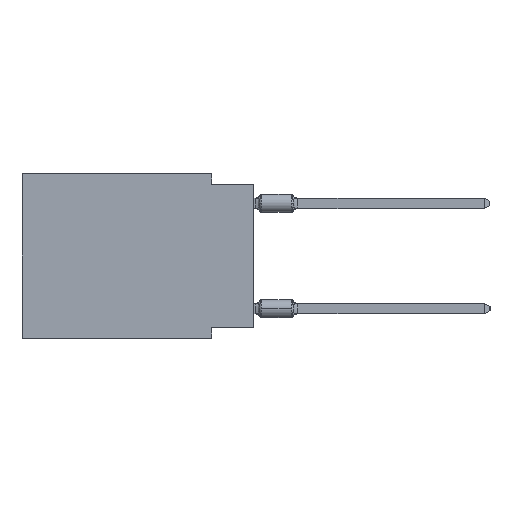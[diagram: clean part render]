
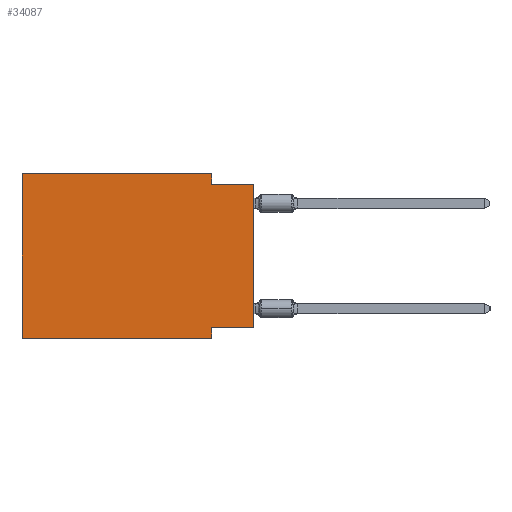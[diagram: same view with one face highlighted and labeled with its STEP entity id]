
A CAD part, left-side view. The second image highlights one B-rep face of the part: STEP entity #34087.
In plain terms, the highlighted planar face has unit normal (-1, 0, 0).
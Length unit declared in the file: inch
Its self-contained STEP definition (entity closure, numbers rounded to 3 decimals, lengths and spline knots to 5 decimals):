
#739 = EDGE_CURVE ( 'NONE', #29654, #5966, #28086, .T. ) ;
#1534 = CARTESIAN_POINT ( 'NONE',  ( 0., 0., -0.025 ) ) ;
#1549 = ORIENTED_EDGE ( 'NONE', *, *, #9261, .F. ) ;
#2342 = CARTESIAN_POINT ( 'NONE',  ( 0., 0.1, -0.39 ) ) ;
#4418 = ORIENTED_EDGE ( 'NONE', *, *, #12862, .T. ) ;
#5966 = VERTEX_POINT ( 'NONE', #20973 ) ;
#7206 = CARTESIAN_POINT ( 'NONE',  ( 0., 0.1, 0. ) ) ;
#8324 = DIRECTION ( 'NONE',  ( 0., -1., 0. ) ) ;
#8336 = VECTOR ( 'NONE', #12207, 39.37008 ) ;
#9104 = CARTESIAN_POINT ( 'NONE',  ( 0., 0.55, 0. ) ) ;
#9261 = EDGE_CURVE ( 'NONE', #26576, #30538, #21467, .T. ) ;
#9269 = CARTESIAN_POINT ( 'NONE',  ( 0., 0.1, -0.365 ) ) ;
#10193 = VERTEX_POINT ( 'NONE', #32350 ) ;
#11018 = LINE ( 'NONE', #14141, #27752 ) ;
#12201 = LINE ( 'NONE', #9104, #18548 ) ;
#12207 = DIRECTION ( 'NONE',  ( 0., 0., 1. ) ) ;
#12862 = EDGE_CURVE ( 'NONE', #26576, #5966, #11018, .T. ) ;
#12966 = VECTOR ( 'NONE', #40085, 39.37008 ) ;
#13892 = VECTOR ( 'NONE', #39950, 39.37008 ) ;
#14141 = CARTESIAN_POINT ( 'NONE',  ( 0., 0.55, -0.39 ) ) ;
#14694 = VERTEX_POINT ( 'NONE', #39168 ) ;
#15979 = CARTESIAN_POINT ( 'NONE',  ( 0., 0.1, 0. ) ) ;
#16192 = DIRECTION ( 'NONE',  ( 0., 0., -1. ) ) ;
#17872 = LINE ( 'NONE', #30564, #12966 ) ;
#18355 = EDGE_CURVE ( 'NONE', #30538, #32892, #12201, .T. ) ;
#18548 = VECTOR ( 'NONE', #37347, 39.37008 ) ;
#18670 = VECTOR ( 'NONE', #36603, 39.37008 ) ;
#19083 = FACE_OUTER_BOUND ( 'NONE', #23932, .T. ) ;
#19933 = VECTOR ( 'NONE', #32557, 39.37008 ) ;
#20973 = CARTESIAN_POINT ( 'NONE',  ( 0., 0.1, -0.39 ) ) ;
#21467 = LINE ( 'NONE', #27296, #13892 ) ;
#23178 = LINE ( 'NONE', #7206, #19933 ) ;
#23932 = EDGE_LOOP ( 'NONE', ( #36011, #37442, #31117, #33733, #1549, #4418, #40938, #29008 ) ) ;
#24119 = LINE ( 'NONE', #1534, #18670 ) ;
#26576 = VERTEX_POINT ( 'NONE', #40420 ) ;
#27207 = AXIS2_PLACEMENT_3D ( 'NONE', #31998, #28055, #16192 ) ;
#27296 = CARTESIAN_POINT ( 'NONE',  ( 0., 0.55, 0. ) ) ;
#27385 = LINE ( 'NONE', #40651, #8336 ) ;
#27752 = VECTOR ( 'NONE', #8324, 39.37008 ) ;
#28055 = DIRECTION ( 'NONE',  ( 1., 0., 0. ) ) ;
#28086 = LINE ( 'NONE', #2342, #35437 ) ;
#28825 = EDGE_CURVE ( 'NONE', #36106, #29654, #17872, .T. ) ;
#29008 = ORIENTED_EDGE ( 'NONE', *, *, #28825, .F. ) ;
#29162 = EDGE_CURVE ( 'NONE', #36106, #14694, #27385, .T. ) ;
#29654 = VERTEX_POINT ( 'NONE', #9269 ) ;
#30538 = VERTEX_POINT ( 'NONE', #37770 ) ;
#30564 = CARTESIAN_POINT ( 'NONE',  ( 0., 0., -0.365 ) ) ;
#31010 = DIRECTION ( 'NONE',  ( 0., 0., -1. ) ) ;
#31117 = ORIENTED_EDGE ( 'NONE', *, *, #34632, .F. ) ;
#31998 = CARTESIAN_POINT ( 'NONE',  ( 0., 0.55, 0. ) ) ;
#32350 = CARTESIAN_POINT ( 'NONE',  ( 0., 0.1, -0.025 ) ) ;
#32557 = DIRECTION ( 'NONE',  ( 0., 0., -1. ) ) ;
#32892 = VERTEX_POINT ( 'NONE', #15979 ) ;
#33733 = ORIENTED_EDGE ( 'NONE', *, *, #18355, .F. ) ;
#34087 = ADVANCED_FACE ( 'NONE', ( #19083 ), #35101, .F. ) ;
#34632 = EDGE_CURVE ( 'NONE', #32892, #10193, #23178, .T. ) ;
#35101 = PLANE ( 'NONE',  #27207 ) ;
#35437 = VECTOR ( 'NONE', #31010, 39.37008 ) ;
#36011 = ORIENTED_EDGE ( 'NONE', *, *, #29162, .T. ) ;
#36106 = VERTEX_POINT ( 'NONE', #40043 ) ;
#36603 = DIRECTION ( 'NONE',  ( 0., -1., 0. ) ) ;
#37347 = DIRECTION ( 'NONE',  ( 0., -1., 0. ) ) ;
#37400 = EDGE_CURVE ( 'NONE', #10193, #14694, #24119, .T. ) ;
#37442 = ORIENTED_EDGE ( 'NONE', *, *, #37400, .F. ) ;
#37770 = CARTESIAN_POINT ( 'NONE',  ( 0., 0.55, 0. ) ) ;
#39168 = CARTESIAN_POINT ( 'NONE',  ( 0., 0., -0.025 ) ) ;
#39950 = DIRECTION ( 'NONE',  ( 0., 0., 1. ) ) ;
#40043 = CARTESIAN_POINT ( 'NONE',  ( 0., 0., -0.365 ) ) ;
#40085 = DIRECTION ( 'NONE',  ( 0., 1., 0. ) ) ;
#40420 = CARTESIAN_POINT ( 'NONE',  ( 0., 0.55, -0.39 ) ) ;
#40651 = CARTESIAN_POINT ( 'NONE',  ( 0., 0., 0. ) ) ;
#40938 = ORIENTED_EDGE ( 'NONE', *, *, #739, .F. ) ;
